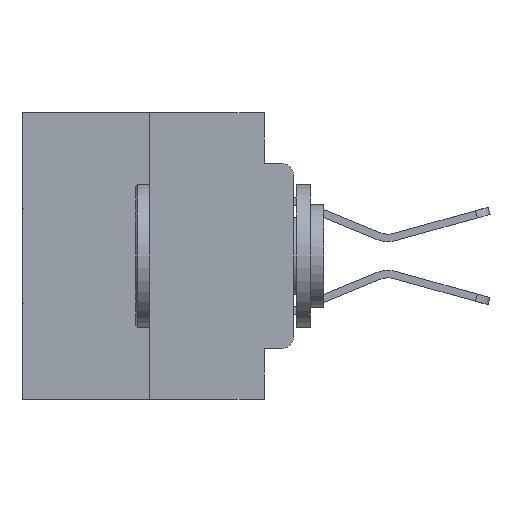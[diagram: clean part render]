
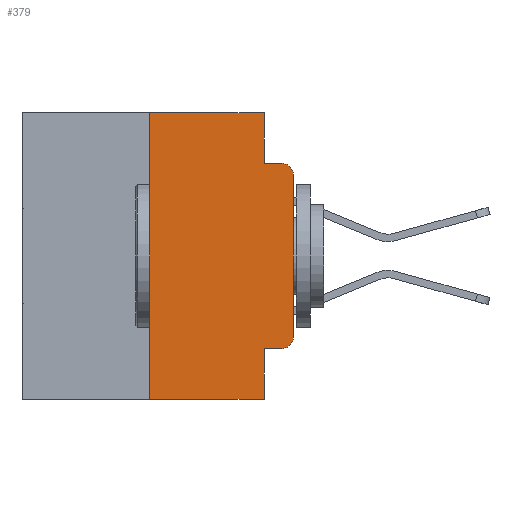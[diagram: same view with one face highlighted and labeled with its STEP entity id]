
A CAD part, left-side view. The second image highlights one B-rep face of the part: STEP entity #379.
In plain terms, the highlighted planar face has unit normal (-1, 0, 0).
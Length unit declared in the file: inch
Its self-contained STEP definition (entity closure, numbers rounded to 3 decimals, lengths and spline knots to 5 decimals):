
#33 = CARTESIAN_POINT ( 'NONE',  ( 0., 0.051, 0. ) ) ;
#92 = EDGE_CURVE ( 'NONE', #16049, #1051, #17057, .T. ) ;
#379 = ADVANCED_FACE ( 'NONE', ( #14604 ), #8019, .F. ) ;
#384 = DIRECTION ( 'NONE',  ( 1., 0., 0. ) ) ;
#1035 = CARTESIAN_POINT ( 'NONE',  ( 0., 0.051, -0.0885 ) ) ;
#1051 = VERTEX_POINT ( 'NONE', #16633 ) ;
#1186 = LINE ( 'NONE', #33, #7280 ) ;
#1308 = CARTESIAN_POINT ( 'NONE',  ( 0., 0.051, -0.4115 ) ) ;
#2730 = VECTOR ( 'NONE', #6258, 39.37008 ) ;
#2925 = VECTOR ( 'NONE', #20003, 39.37008 ) ;
#3221 = ORIENTED_EDGE ( 'NONE', *, *, #9321, .T. ) ;
#3254 = EDGE_CURVE ( 'NONE', #4504, #16000, #14130, .T. ) ;
#4017 = EDGE_CURVE ( 'NONE', #24477, #9378, #6072, .T. ) ;
#4504 = VERTEX_POINT ( 'NONE', #1035 ) ;
#4798 = EDGE_CURVE ( 'NONE', #1051, #16000, #14716, .T. ) ;
#5636 = LINE ( 'NONE', #22776, #16761 ) ;
#6072 = LINE ( 'NONE', #23957, #17203 ) ;
#6258 = DIRECTION ( 'NONE',  ( 0., -1., 0. ) ) ;
#6307 = EDGE_CURVE ( 'NONE', #8155, #24477, #5636, .T. ) ;
#6599 = CARTESIAN_POINT ( 'NONE',  ( 0., 0.02, -0.3915 ) ) ;
#7121 = ORIENTED_EDGE ( 'NONE', *, *, #4017, .F. ) ;
#7209 = DIRECTION ( 'NONE',  ( 0., 0., -1. ) ) ;
#7255 = CARTESIAN_POINT ( 'NONE',  ( 0., 0.02, -0.0885 ) ) ;
#7280 = VECTOR ( 'NONE', #13610, 39.37008 ) ;
#7802 = EDGE_CURVE ( 'NONE', #9378, #4504, #1186, .T. ) ;
#8019 = PLANE ( 'NONE',  #23844 ) ;
#8155 = VERTEX_POINT ( 'NONE', #23554 ) ;
#8306 = CIRCLE ( 'NONE', #23713, 0.02 ) ;
#8480 = DIRECTION ( 'NONE',  ( 0., -1., 0. ) ) ;
#8554 = ORIENTED_EDGE ( 'NONE', *, *, #12280, .F. ) ;
#8869 = DIRECTION ( 'NONE',  ( 0., 0., -1. ) ) ;
#9321 = EDGE_CURVE ( 'NONE', #15142, #22108, #10375, .T. ) ;
#9378 = VERTEX_POINT ( 'NONE', #23791 ) ;
#9479 = CARTESIAN_POINT ( 'NONE',  ( 0., 0.051, -0.4115 ) ) ;
#9587 = ORIENTED_EDGE ( 'NONE', *, *, #4798, .T. ) ;
#9727 = CARTESIAN_POINT ( 'NONE',  ( 0., 0.02, -0.4115 ) ) ;
#10375 = LINE ( 'NONE', #1308, #16241 ) ;
#10618 = AXIS2_PLACEMENT_3D ( 'NONE', #26595, #13375, #28759 ) ;
#11301 = DIRECTION ( 'NONE',  ( 0., 0., -1. ) ) ;
#11868 = VECTOR ( 'NONE', #21261, 39.37008 ) ;
#11938 = CARTESIAN_POINT ( 'NONE',  ( 0., 0., -0.3915 ) ) ;
#12280 = EDGE_CURVE ( 'NONE', #15142, #16131, #12557, .T. ) ;
#12557 = LINE ( 'NONE', #26709, #22941 ) ;
#13375 = DIRECTION ( 'NONE',  ( -1., 0., 0. ) ) ;
#13610 = DIRECTION ( 'NONE',  ( 0., 0., -1. ) ) ;
#13753 = EDGE_CURVE ( 'NONE', #22108, #16049, #8306, .T. ) ;
#14070 = EDGE_LOOP ( 'NONE', ( #20664, #9587, #22049, #23412, #7121, #18944, #19647, #8554, #3221, #22400 ) ) ;
#14130 = LINE ( 'NONE', #19968, #2925 ) ;
#14604 = FACE_OUTER_BOUND ( 'NONE', #14070, .T. ) ;
#14716 = CIRCLE ( 'NONE', #10618, 0.02 ) ;
#14799 = DIRECTION ( 'NONE',  ( 0., -1., 0. ) ) ;
#15142 = VERTEX_POINT ( 'NONE', #9479 ) ;
#16000 = VERTEX_POINT ( 'NONE', #7255 ) ;
#16045 = LINE ( 'NONE', #21792, #2730 ) ;
#16049 = VERTEX_POINT ( 'NONE', #11938 ) ;
#16131 = VERTEX_POINT ( 'NONE', #23234 ) ;
#16241 = VECTOR ( 'NONE', #14799, 39.37008 ) ;
#16352 = EDGE_CURVE ( 'NONE', #8155, #16131, #16045, .T. ) ;
#16633 = CARTESIAN_POINT ( 'NONE',  ( 0., 0., -0.1085 ) ) ;
#16761 = VECTOR ( 'NONE', #27175, 39.37008 ) ;
#17057 = LINE ( 'NONE', #21165, #11868 ) ;
#17203 = VECTOR ( 'NONE', #8480, 39.37008 ) ;
#18352 = CARTESIAN_POINT ( 'NONE',  ( 0., 0.25, 0. ) ) ;
#18944 = ORIENTED_EDGE ( 'NONE', *, *, #6307, .F. ) ;
#19647 = ORIENTED_EDGE ( 'NONE', *, *, #16352, .T. ) ;
#19968 = CARTESIAN_POINT ( 'NONE',  ( 0., 0.051, -0.0885 ) ) ;
#20003 = DIRECTION ( 'NONE',  ( 0., -1., 0. ) ) ;
#20419 = CARTESIAN_POINT ( 'NONE',  ( 0., 0.473, 0. ) ) ;
#20664 = ORIENTED_EDGE ( 'NONE', *, *, #92, .T. ) ;
#21165 = CARTESIAN_POINT ( 'NONE',  ( 0., 0., 0. ) ) ;
#21261 = DIRECTION ( 'NONE',  ( 0., 0., 1. ) ) ;
#21792 = CARTESIAN_POINT ( 'NONE',  ( 0., 0.473, -0.5 ) ) ;
#22049 = ORIENTED_EDGE ( 'NONE', *, *, #3254, .F. ) ;
#22108 = VERTEX_POINT ( 'NONE', #9727 ) ;
#22127 = DIRECTION ( 'NONE',  ( -1., 0., 0. ) ) ;
#22400 = ORIENTED_EDGE ( 'NONE', *, *, #13753, .T. ) ;
#22776 = CARTESIAN_POINT ( 'NONE',  ( 0., 0.25, 0. ) ) ;
#22941 = VECTOR ( 'NONE', #11301, 39.37008 ) ;
#23234 = CARTESIAN_POINT ( 'NONE',  ( 0., 0.051, -0.5 ) ) ;
#23412 = ORIENTED_EDGE ( 'NONE', *, *, #7802, .F. ) ;
#23554 = CARTESIAN_POINT ( 'NONE',  ( 0., 0.25, -0.5 ) ) ;
#23713 = AXIS2_PLACEMENT_3D ( 'NONE', #6599, #22127, #8869 ) ;
#23791 = CARTESIAN_POINT ( 'NONE',  ( 0., 0.051, 0. ) ) ;
#23844 = AXIS2_PLACEMENT_3D ( 'NONE', #20419, #384, #7209 ) ;
#23957 = CARTESIAN_POINT ( 'NONE',  ( 0., 0.473, 0. ) ) ;
#24477 = VERTEX_POINT ( 'NONE', #18352 ) ;
#26595 = CARTESIAN_POINT ( 'NONE',  ( 0., 0.02, -0.1085 ) ) ;
#26709 = CARTESIAN_POINT ( 'NONE',  ( 0., 0.051, 0. ) ) ;
#27175 = DIRECTION ( 'NONE',  ( 0., 0., 1. ) ) ;
#28759 = DIRECTION ( 'NONE',  ( 0., 0., -1. ) ) ;
